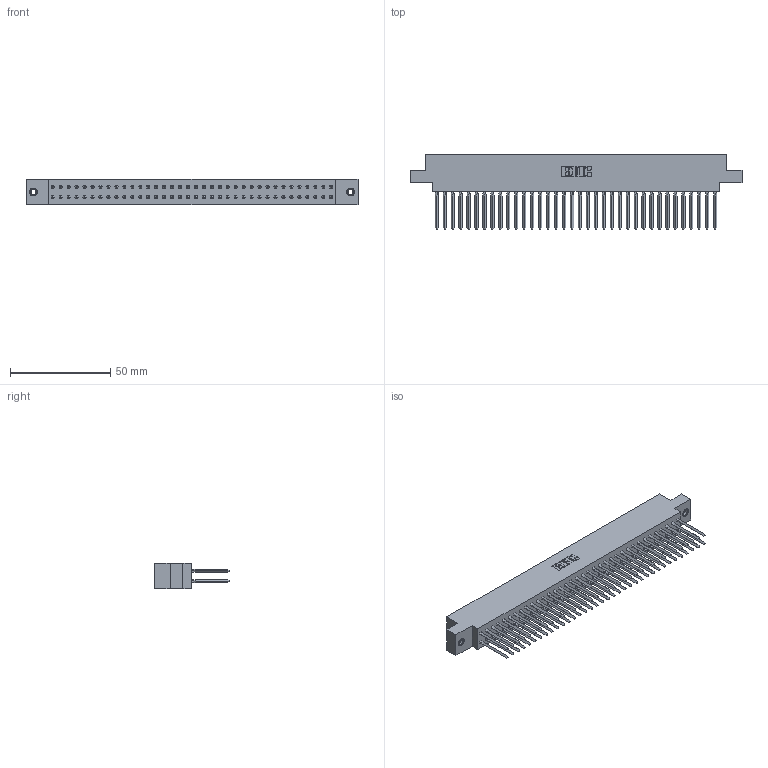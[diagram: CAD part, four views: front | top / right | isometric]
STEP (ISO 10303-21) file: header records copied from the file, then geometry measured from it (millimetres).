
FILE_DESCRIPTION (( 'STEP AP203' ), '1' );
FILE_NAME ('317-072-542-807.STEP', '2020-02-28T07:34:20', ( '' ), ( '' ), 'SwSTEP 2.0', 'SolidWorks 2016', '' );
FILE_SCHEMA (( 'CONFIG_CONTROL_DESIGN' ));
Length unit declared in the file: inch
Products named in the file (4): 317 Part_.156 Dia - TI; 345-250-001_345-250-005-103; 317-072-542-807; 317-290-003_542
Assembly tree (75 placements, depth 2):
  317-072-542-807
    317 Part_.156 Dia - TI
    317-290-003_542  x72
    345-250-001_345-250-005-103  x2
Bounding box: 165.35 x 37.34 x 12.7 mm (x, y, z)
Volume: 26873 mm3; surface area: 37213.2 mm2
Topology: 75 solids, 75 shells, 4266 faces, 11931 edges, 7610 vertices
Faces by surface type: plane 3402, cylinder 560, bspline 288, cone 12, torus 4
Entity records: 53078 total; most frequent: CARTESIAN_POINT 9480, ORIENTED_EDGE 9136, DIRECTION 7734, EDGE_CURVE 4568, VECTOR 4378, LINE 4378, VERTEX_POINT 3036, AXIS2_PLACEMENT_3D 1678
